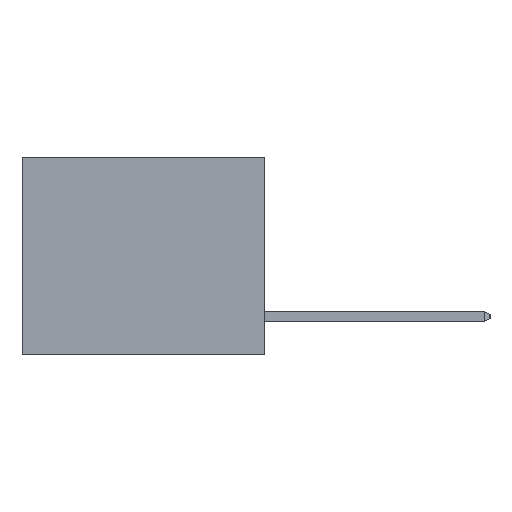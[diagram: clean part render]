
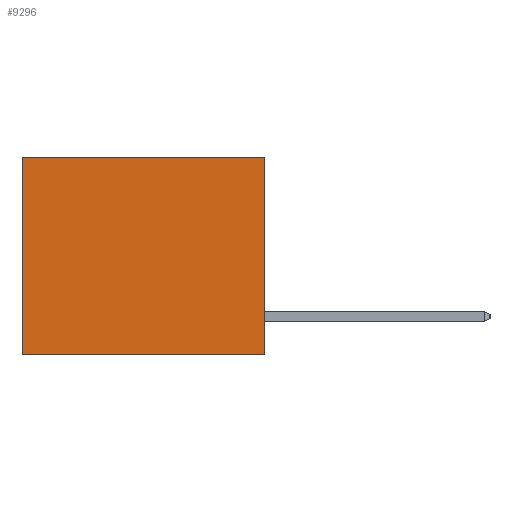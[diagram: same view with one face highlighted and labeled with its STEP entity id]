
A CAD part, left-side view. The second image highlights one B-rep face of the part: STEP entity #9296.
In plain terms, the highlighted planar face has unit normal (-1, 0, 0).
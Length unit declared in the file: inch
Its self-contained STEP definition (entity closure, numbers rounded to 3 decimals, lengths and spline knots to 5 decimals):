
#108 = ORIENTED_EDGE ( 'NONE', *, *, #8505, .F. ) ;
#182 = CARTESIAN_POINT ( 'NONE',  ( 0.3165, 0.6, -0.49 ) ) ;
#297 = VECTOR ( 'NONE', #3373, 39.37008 ) ;
#688 = DIRECTION ( 'NONE',  ( 0., 0., -1. ) ) ;
#1554 = CARTESIAN_POINT ( 'NONE',  ( 0.3165, 0., -0.49 ) ) ;
#2056 = VERTEX_POINT ( 'NONE', #10152 ) ;
#2336 = VECTOR ( 'NONE', #2796, 39.37008 ) ;
#2796 = DIRECTION ( 'NONE',  ( 0., 0., -1. ) ) ;
#3215 = CARTESIAN_POINT ( 'NONE',  ( 0.3165, 0., -0.49 ) ) ;
#3373 = DIRECTION ( 'NONE',  ( 0., 1., 0. ) ) ;
#3728 = DIRECTION ( 'NONE',  ( 1., 0., 0. ) ) ;
#4680 = VERTEX_POINT ( 'NONE', #182 ) ;
#5467 = AXIS2_PLACEMENT_3D ( 'NONE', #14313, #3728, #9741 ) ;
#6284 = EDGE_CURVE ( 'NONE', #12662, #4680, #12720, .T. ) ;
#6755 = ORIENTED_EDGE ( 'NONE', *, *, #12236, .T. ) ;
#6799 = LINE ( 'NONE', #14853, #11455 ) ;
#8304 = CARTESIAN_POINT ( 'NONE',  ( 0.3165, 0., -0.49 ) ) ;
#8505 = EDGE_CURVE ( 'NONE', #14840, #12662, #10521, .T. ) ;
#8996 = CARTESIAN_POINT ( 'NONE',  ( 0.3165, 0., 0. ) ) ;
#9296 = ADVANCED_FACE ( 'NONE', ( #13159 ), #14409, .F. ) ;
#9741 = DIRECTION ( 'NONE',  ( 0., 0., -1. ) ) ;
#9806 = ORIENTED_EDGE ( 'NONE', *, *, #9979, .T. ) ;
#9979 = EDGE_CURVE ( 'NONE', #2056, #4680, #6799, .T. ) ;
#10152 = CARTESIAN_POINT ( 'NONE',  ( 0.3165, 0.6, 0. ) ) ;
#10464 = ORIENTED_EDGE ( 'NONE', *, *, #6284, .F. ) ;
#10521 = LINE ( 'NONE', #1554, #2336 ) ;
#10710 = LINE ( 'NONE', #13926, #297 ) ;
#11408 = DIRECTION ( 'NONE',  ( 0., 1., 0. ) ) ;
#11455 = VECTOR ( 'NONE', #688, 39.37008 ) ;
#12236 = EDGE_CURVE ( 'NONE', #14840, #2056, #10710, .T. ) ;
#12662 = VERTEX_POINT ( 'NONE', #8304 ) ;
#12720 = LINE ( 'NONE', #3215, #13987 ) ;
#13159 = FACE_OUTER_BOUND ( 'NONE', #13690, .T. ) ;
#13690 = EDGE_LOOP ( 'NONE', ( #9806, #10464, #108, #6755 ) ) ;
#13926 = CARTESIAN_POINT ( 'NONE',  ( 0.3165, 0., 0. ) ) ;
#13987 = VECTOR ( 'NONE', #11408, 39.37008 ) ;
#14313 = CARTESIAN_POINT ( 'NONE',  ( 0.3165, 0., -0.49 ) ) ;
#14409 = PLANE ( 'NONE',  #5467 ) ;
#14840 = VERTEX_POINT ( 'NONE', #8996 ) ;
#14853 = CARTESIAN_POINT ( 'NONE',  ( 0.3165, 0.6, -0.49 ) ) ;
